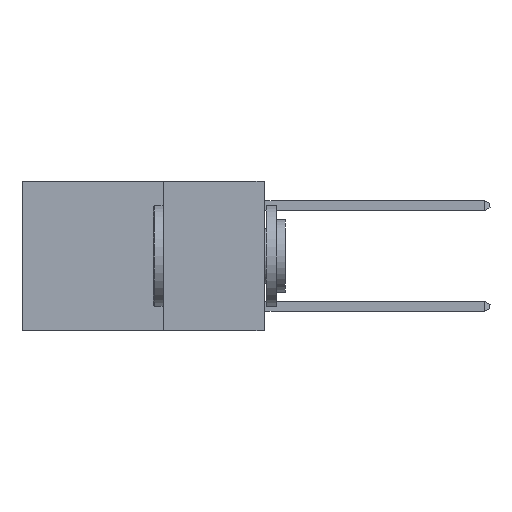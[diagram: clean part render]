
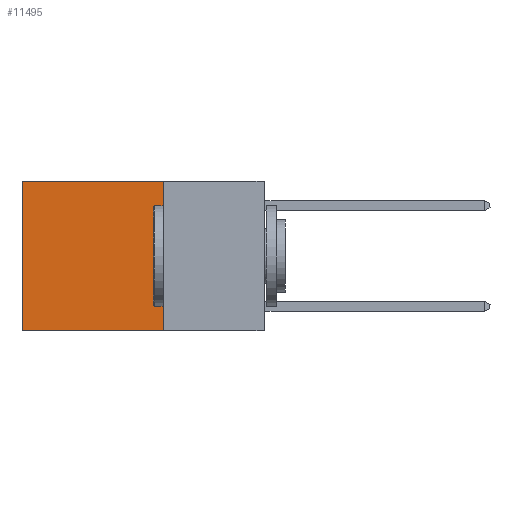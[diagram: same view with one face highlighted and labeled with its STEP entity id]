
A CAD part, left-side view. The second image highlights one B-rep face of the part: STEP entity #11495.
In plain terms, the highlighted planar face has unit normal (-1, 0, 0).
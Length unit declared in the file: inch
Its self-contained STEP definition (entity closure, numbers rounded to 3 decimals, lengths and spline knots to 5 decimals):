
#314 = EDGE_CURVE ( 'NONE', #1598, #10303, #10214, .T. ) ;
#427 = CARTESIAN_POINT ( 'NONE',  ( 0.2625, 0.6, 0. ) ) ;
#586 = ORIENTED_EDGE ( 'NONE', *, *, #3513, .T. ) ;
#850 = CARTESIAN_POINT ( 'NONE',  ( 0.2625, 0.25, -0.37 ) ) ;
#1101 = DIRECTION ( 'NONE',  ( 0., 0., -1. ) ) ;
#1598 = VERTEX_POINT ( 'NONE', #9323 ) ;
#1971 = DIRECTION ( 'NONE',  ( 0., 1., 0. ) ) ;
#2118 = EDGE_LOOP ( 'NONE', ( #586, #2265, #7524, #3769 ) ) ;
#2265 = ORIENTED_EDGE ( 'NONE', *, *, #10008, .F. ) ;
#2797 = DIRECTION ( 'NONE',  ( 1., 0., 0. ) ) ;
#3008 = CARTESIAN_POINT ( 'NONE',  ( 0.2625, 0.25, 0. ) ) ;
#3416 = LINE ( 'NONE', #427, #11702 ) ;
#3513 = EDGE_CURVE ( 'NONE', #10303, #5581, #3416, .T. ) ;
#3769 = ORIENTED_EDGE ( 'NONE', *, *, #314, .T. ) ;
#4622 = PLANE ( 'NONE',  #5978 ) ;
#4670 = LINE ( 'NONE', #3008, #5816 ) ;
#5581 = VERTEX_POINT ( 'NONE', #10336 ) ;
#5740 = CARTESIAN_POINT ( 'NONE',  ( 0.2625, 0.6, 0. ) ) ;
#5816 = VECTOR ( 'NONE', #1101, 39.37008 ) ;
#5978 = AXIS2_PLACEMENT_3D ( 'NONE', #7419, #2797, #8290 ) ;
#6270 = LINE ( 'NONE', #11746, #6730 ) ;
#6414 = EDGE_CURVE ( 'NONE', #1598, #11461, #4670, .T. ) ;
#6730 = VECTOR ( 'NONE', #10930, 39.37008 ) ;
#6983 = FACE_OUTER_BOUND ( 'NONE', #2118, .T. ) ;
#7419 = CARTESIAN_POINT ( 'NONE',  ( 0.2625, 0.25, 0. ) ) ;
#7524 = ORIENTED_EDGE ( 'NONE', *, *, #6414, .F. ) ;
#7576 = CARTESIAN_POINT ( 'NONE',  ( 0.2625, 0.25, 0. ) ) ;
#8290 = DIRECTION ( 'NONE',  ( 0., 0., -1. ) ) ;
#9323 = CARTESIAN_POINT ( 'NONE',  ( 0.2625, 0.25, 0. ) ) ;
#10008 = EDGE_CURVE ( 'NONE', #11461, #5581, #6270, .T. ) ;
#10214 = LINE ( 'NONE', #7576, #11359 ) ;
#10303 = VERTEX_POINT ( 'NONE', #5740 ) ;
#10336 = CARTESIAN_POINT ( 'NONE',  ( 0.2625, 0.6, -0.37 ) ) ;
#10526 = DIRECTION ( 'NONE',  ( 0., 0., -1. ) ) ;
#10930 = DIRECTION ( 'NONE',  ( 0., 1., 0. ) ) ;
#11359 = VECTOR ( 'NONE', #1971, 39.37008 ) ;
#11461 = VERTEX_POINT ( 'NONE', #850 ) ;
#11495 = ADVANCED_FACE ( 'NONE', ( #6983 ), #4622, .F. ) ;
#11702 = VECTOR ( 'NONE', #10526, 39.37008 ) ;
#11746 = CARTESIAN_POINT ( 'NONE',  ( 0.2625, 0.25, -0.37 ) ) ;
